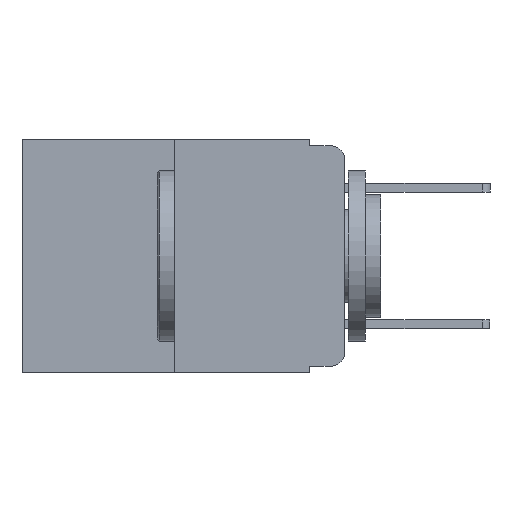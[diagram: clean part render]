
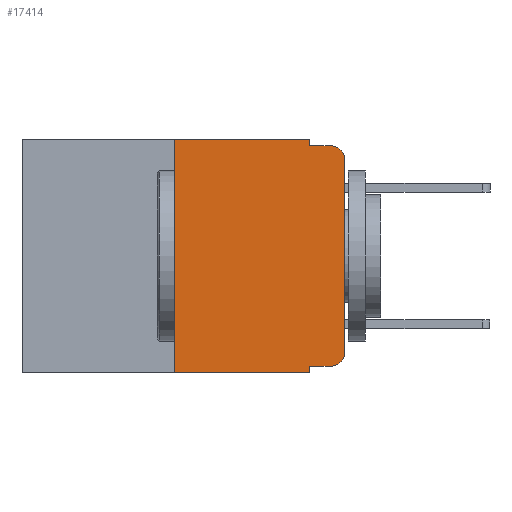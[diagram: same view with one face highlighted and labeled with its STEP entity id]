
A CAD part, left-side view. The second image highlights one B-rep face of the part: STEP entity #17414.
In plain terms, the highlighted planar face has unit normal (-1, 0, 0).
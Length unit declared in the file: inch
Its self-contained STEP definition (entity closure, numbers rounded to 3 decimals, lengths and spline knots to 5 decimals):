
#489 = EDGE_CURVE ( 'NONE', #5905, #18145, #6254, .T. ) ;
#652 = LINE ( 'NONE', #23396, #5117 ) ;
#1059 = CARTESIAN_POINT ( 'NONE',  ( 0., 0.051, -0.333 ) ) ;
#1060 = DIRECTION ( 'NONE',  ( 0., 0., -1. ) ) ;
#1066 = VERTEX_POINT ( 'NONE', #20263 ) ;
#1211 = VERTEX_POINT ( 'NONE', #18499 ) ;
#1459 = VERTEX_POINT ( 'NONE', #3675 ) ;
#2167 = CARTESIAN_POINT ( 'NONE',  ( 0., 0.051, 0. ) ) ;
#3303 = ORIENTED_EDGE ( 'NONE', *, *, #18024, .T. ) ;
#3635 = CIRCLE ( 'NONE', #11937, 0.02 ) ;
#3675 = CARTESIAN_POINT ( 'NONE',  ( 0., 0.051, -0.343 ) ) ;
#4062 = EDGE_CURVE ( 'NONE', #1066, #17049, #17639, .T. ) ;
#4452 = CARTESIAN_POINT ( 'NONE',  ( 0., 0.051, 0. ) ) ;
#4613 = CIRCLE ( 'NONE', #19651, 0.02 ) ;
#4635 = VECTOR ( 'NONE', #16107, 39.37008 ) ;
#4743 = CARTESIAN_POINT ( 'NONE',  ( 0., 0.473, 0. ) ) ;
#4966 = ORIENTED_EDGE ( 'NONE', *, *, #489, .T. ) ;
#5117 = VECTOR ( 'NONE', #14681, 39.37008 ) ;
#5905 = VERTEX_POINT ( 'NONE', #1059 ) ;
#6138 = EDGE_CURVE ( 'NONE', #20034, #8427, #22684, .T. ) ;
#6244 = ORIENTED_EDGE ( 'NONE', *, *, #6138, .T. ) ;
#6254 = LINE ( 'NONE', #15323, #9944 ) ;
#6434 = ORIENTED_EDGE ( 'NONE', *, *, #12344, .T. ) ;
#6649 = DIRECTION ( 'NONE',  ( -1., 0., 0. ) ) ;
#6779 = DIRECTION ( 'NONE',  ( 0., -1., 0. ) ) ;
#7580 = ORIENTED_EDGE ( 'NONE', *, *, #9920, .F. ) ;
#8427 = VERTEX_POINT ( 'NONE', #11960 ) ;
#8444 = PLANE ( 'NONE',  #9202 ) ;
#8719 = CARTESIAN_POINT ( 'NONE',  ( 0., 0.02, -0.333 ) ) ;
#8990 = LINE ( 'NONE', #16160, #18572 ) ;
#9120 = DIRECTION ( 'NONE',  ( 0., 0., 1. ) ) ;
#9202 = AXIS2_PLACEMENT_3D ( 'NONE', #4743, #10249, #22649 ) ;
#9920 = EDGE_CURVE ( 'NONE', #13637, #1211, #8990, .T. ) ;
#9944 = VECTOR ( 'NONE', #18503, 39.37008 ) ;
#9980 = CARTESIAN_POINT ( 'NONE',  ( 0., 0., -0.313 ) ) ;
#10048 = ORIENTED_EDGE ( 'NONE', *, *, #11749, .T. ) ;
#10249 = DIRECTION ( 'NONE',  ( 1., 0., 0. ) ) ;
#10943 = CARTESIAN_POINT ( 'NONE',  ( 0., 0., 0. ) ) ;
#11749 = EDGE_CURVE ( 'NONE', #1066, #1459, #12335, .T. ) ;
#11807 = ORIENTED_EDGE ( 'NONE', *, *, #4062, .F. ) ;
#11883 = EDGE_CURVE ( 'NONE', #17049, #15665, #23083, .T. ) ;
#11937 = AXIS2_PLACEMENT_3D ( 'NONE', #17494, #6649, #19249 ) ;
#11960 = CARTESIAN_POINT ( 'NONE',  ( 0., 0., -0.03 ) ) ;
#12135 = DIRECTION ( 'NONE',  ( -1., 0., 0. ) ) ;
#12335 = LINE ( 'NONE', #19372, #21243 ) ;
#12344 = EDGE_CURVE ( 'NONE', #8427, #1211, #4613, .T. ) ;
#12534 = CARTESIAN_POINT ( 'NONE',  ( 0., 0.473, 0. ) ) ;
#12953 = VECTOR ( 'NONE', #17190, 39.37008 ) ;
#13637 = VERTEX_POINT ( 'NONE', #21708 ) ;
#13642 = EDGE_CURVE ( 'NONE', #5905, #1459, #652, .T. ) ;
#14006 = EDGE_LOOP ( 'NONE', ( #6244, #6434, #7580, #18065, #15593, #11807, #10048, #17509, #4966, #3303 ) ) ;
#14681 = DIRECTION ( 'NONE',  ( 0., 0., -1. ) ) ;
#15323 = CARTESIAN_POINT ( 'NONE',  ( 0., 0.051, -0.333 ) ) ;
#15356 = DIRECTION ( 'NONE',  ( 0., 0., 1. ) ) ;
#15593 = ORIENTED_EDGE ( 'NONE', *, *, #11883, .F. ) ;
#15665 = VERTEX_POINT ( 'NONE', #2167 ) ;
#15700 = CARTESIAN_POINT ( 'NONE',  ( 0., 0.25, 0. ) ) ;
#16107 = DIRECTION ( 'NONE',  ( 0., -1., 0. ) ) ;
#16160 = CARTESIAN_POINT ( 'NONE',  ( 0., 0.051, -0.01 ) ) ;
#17049 = VERTEX_POINT ( 'NONE', #23256 ) ;
#17190 = DIRECTION ( 'NONE',  ( 0., 0., -1. ) ) ;
#17414 = ADVANCED_FACE ( 'NONE', ( #23021 ), #8444, .F. ) ;
#17494 = CARTESIAN_POINT ( 'NONE',  ( 0., 0.02, -0.313 ) ) ;
#17509 = ORIENTED_EDGE ( 'NONE', *, *, #13642, .F. ) ;
#17639 = LINE ( 'NONE', #15700, #21706 ) ;
#18024 = EDGE_CURVE ( 'NONE', #18145, #20034, #3635, .T. ) ;
#18065 = ORIENTED_EDGE ( 'NONE', *, *, #20016, .F. ) ;
#18085 = VECTOR ( 'NONE', #9120, 39.37008 ) ;
#18145 = VERTEX_POINT ( 'NONE', #8719 ) ;
#18299 = LINE ( 'NONE', #4452, #12953 ) ;
#18499 = CARTESIAN_POINT ( 'NONE',  ( 0., 0.02, -0.01 ) ) ;
#18503 = DIRECTION ( 'NONE',  ( 0., -1., 0. ) ) ;
#18572 = VECTOR ( 'NONE', #23151, 39.37008 ) ;
#19249 = DIRECTION ( 'NONE',  ( 0., 0., -1. ) ) ;
#19372 = CARTESIAN_POINT ( 'NONE',  ( 0., 0.473, -0.343 ) ) ;
#19651 = AXIS2_PLACEMENT_3D ( 'NONE', #22717, #12135, #1060 ) ;
#20016 = EDGE_CURVE ( 'NONE', #15665, #13637, #18299, .T. ) ;
#20034 = VERTEX_POINT ( 'NONE', #9980 ) ;
#20263 = CARTESIAN_POINT ( 'NONE',  ( 0., 0.25, -0.343 ) ) ;
#21243 = VECTOR ( 'NONE', #6779, 39.37008 ) ;
#21706 = VECTOR ( 'NONE', #15356, 39.37008 ) ;
#21708 = CARTESIAN_POINT ( 'NONE',  ( 0., 0.051, -0.01 ) ) ;
#22649 = DIRECTION ( 'NONE',  ( 0., 0., -1. ) ) ;
#22684 = LINE ( 'NONE', #10943, #18085 ) ;
#22717 = CARTESIAN_POINT ( 'NONE',  ( 0., 0.02, -0.03 ) ) ;
#23021 = FACE_OUTER_BOUND ( 'NONE', #14006, .T. ) ;
#23083 = LINE ( 'NONE', #12534, #4635 ) ;
#23151 = DIRECTION ( 'NONE',  ( 0., -1., 0. ) ) ;
#23256 = CARTESIAN_POINT ( 'NONE',  ( 0., 0.25, 0. ) ) ;
#23396 = CARTESIAN_POINT ( 'NONE',  ( 0., 0.051, 0. ) ) ;
